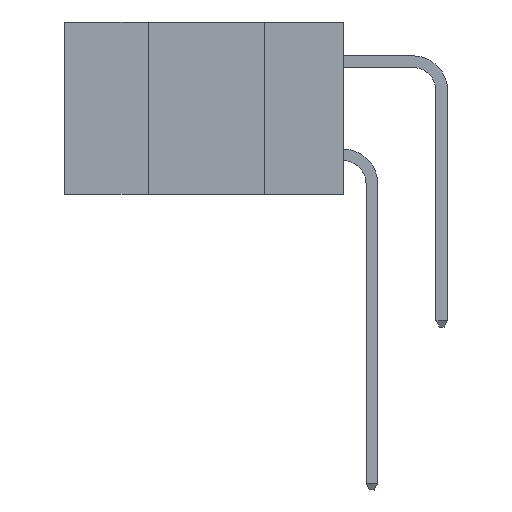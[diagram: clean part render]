
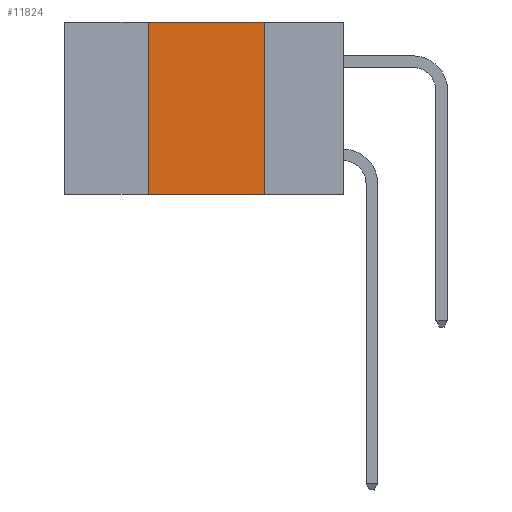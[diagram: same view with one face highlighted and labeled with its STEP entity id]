
A CAD part, left-side view. The second image highlights one B-rep face of the part: STEP entity #11824.
In plain terms, the highlighted planar face has unit normal (-1, 0, 0).
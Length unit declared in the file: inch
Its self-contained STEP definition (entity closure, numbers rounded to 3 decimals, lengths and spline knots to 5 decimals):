
#53 = EDGE_CURVE ( 'NONE', #462, #6559, #10373, .T. ) ;
#252 = CARTESIAN_POINT ( 'NONE',  ( 0., 0.17, -0.37 ) ) ;
#462 = VERTEX_POINT ( 'NONE', #3380 ) ;
#775 = LINE ( 'NONE', #11632, #1369 ) ;
#1134 = ORIENTED_EDGE ( 'NONE', *, *, #7185, .F. ) ;
#1369 = VECTOR ( 'NONE', #4864, 39.37008 ) ;
#1882 = FACE_OUTER_BOUND ( 'NONE', #5377, .T. ) ;
#2145 = VECTOR ( 'NONE', #10195, 39.37008 ) ;
#2414 = CARTESIAN_POINT ( 'NONE',  ( 0., 0.17, 0. ) ) ;
#2905 = ORIENTED_EDGE ( 'NONE', *, *, #8095, .F. ) ;
#2953 = VECTOR ( 'NONE', #11517, 39.37008 ) ;
#3253 = DIRECTION ( 'NONE',  ( 0., -1., 0. ) ) ;
#3292 = EDGE_CURVE ( 'NONE', #3448, #7700, #8084, .T. ) ;
#3380 = CARTESIAN_POINT ( 'NONE',  ( 0., 0.42, -0.37 ) ) ;
#3448 = VERTEX_POINT ( 'NONE', #6939 ) ;
#3456 = VECTOR ( 'NONE', #3253, 39.37008 ) ;
#3706 = CARTESIAN_POINT ( 'NONE',  ( 0., 0.6, 0. ) ) ;
#4864 = DIRECTION ( 'NONE',  ( 0., 0., 1. ) ) ;
#5377 = EDGE_LOOP ( 'NONE', ( #1134, #6687, #2905, #5957 ) ) ;
#5904 = LINE ( 'NONE', #2414, #2145 ) ;
#5957 = ORIENTED_EDGE ( 'NONE', *, *, #53, .T. ) ;
#6554 = PLANE ( 'NONE',  #8089 ) ;
#6559 = VERTEX_POINT ( 'NONE', #252 ) ;
#6687 = ORIENTED_EDGE ( 'NONE', *, *, #3292, .F. ) ;
#6814 = CARTESIAN_POINT ( 'NONE',  ( 0., 0.6, 0. ) ) ;
#6939 = CARTESIAN_POINT ( 'NONE',  ( 0., 0.42, 0. ) ) ;
#7038 = CARTESIAN_POINT ( 'NONE',  ( 0., 0.17, 0. ) ) ;
#7072 = CARTESIAN_POINT ( 'NONE',  ( 0., 0.6, -0.37 ) ) ;
#7185 = EDGE_CURVE ( 'NONE', #7700, #6559, #5904, .T. ) ;
#7700 = VERTEX_POINT ( 'NONE', #7038 ) ;
#8084 = LINE ( 'NONE', #6814, #2953 ) ;
#8089 = AXIS2_PLACEMENT_3D ( 'NONE', #3706, #9774, #10619 ) ;
#8095 = EDGE_CURVE ( 'NONE', #462, #3448, #775, .T. ) ;
#9774 = DIRECTION ( 'NONE',  ( 1., 0., 0. ) ) ;
#10195 = DIRECTION ( 'NONE',  ( 0., 0., -1. ) ) ;
#10373 = LINE ( 'NONE', #7072, #3456 ) ;
#10619 = DIRECTION ( 'NONE',  ( 0., 0., -1. ) ) ;
#11517 = DIRECTION ( 'NONE',  ( 0., -1., 0. ) ) ;
#11632 = CARTESIAN_POINT ( 'NONE',  ( 0., 0.42, 0. ) ) ;
#11824 = ADVANCED_FACE ( 'NONE', ( #1882 ), #6554, .F. ) ;
